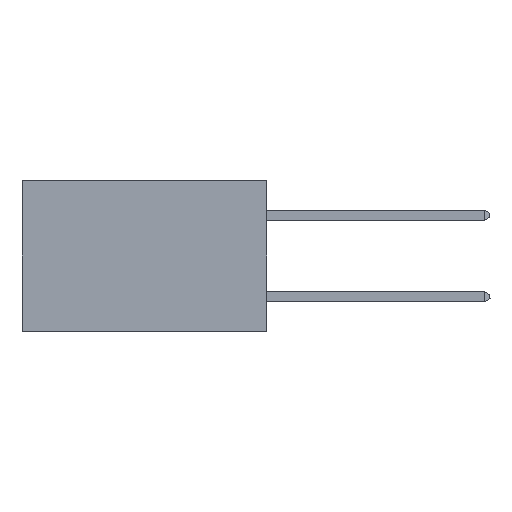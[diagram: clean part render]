
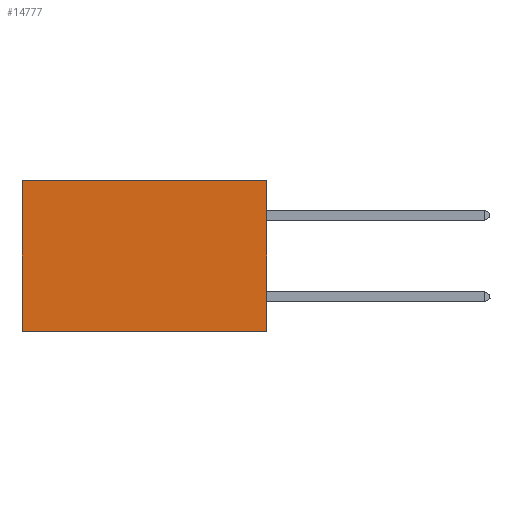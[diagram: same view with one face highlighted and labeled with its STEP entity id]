
A CAD part, left-side view. The second image highlights one B-rep face of the part: STEP entity #14777.
In plain terms, the highlighted planar face has unit normal (-1, 0, 0).
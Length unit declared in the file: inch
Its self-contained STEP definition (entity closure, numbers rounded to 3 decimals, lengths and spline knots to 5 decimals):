
#618 = ORIENTED_EDGE ( 'NONE', *, *, #17312, .T. ) ;
#1189 = VECTOR ( 'NONE', #5908, 39.37008 ) ;
#1414 = CARTESIAN_POINT ( 'NONE',  ( 0.2875, 0.6, 0. ) ) ;
#3554 = VERTEX_POINT ( 'NONE', #24488 ) ;
#5908 = DIRECTION ( 'NONE',  ( 0., 1., 0. ) ) ;
#6450 = FACE_OUTER_BOUND ( 'NONE', #19353, .T. ) ;
#6460 = AXIS2_PLACEMENT_3D ( 'NONE', #15453, #22095, #24395 ) ;
#6669 = LINE ( 'NONE', #29387, #25458 ) ;
#7198 = ORIENTED_EDGE ( 'NONE', *, *, #25629, .T. ) ;
#7609 = VERTEX_POINT ( 'NONE', #23046 ) ;
#7799 = EDGE_CURVE ( 'NONE', #15069, #3554, #20726, .T. ) ;
#9497 = VECTOR ( 'NONE', #23343, 39.37008 ) ;
#10221 = LINE ( 'NONE', #22847, #9497 ) ;
#14090 = DIRECTION ( 'NONE',  ( 0., 0., -1. ) ) ;
#14777 = ADVANCED_FACE ( 'NONE', ( #6450 ), #29092, .F. ) ;
#15069 = VERTEX_POINT ( 'NONE', #26815 ) ;
#15453 = CARTESIAN_POINT ( 'NONE',  ( 0.2875, 0., 0. ) ) ;
#17312 = EDGE_CURVE ( 'NONE', #15069, #22805, #10221, .T. ) ;
#17815 = DIRECTION ( 'NONE',  ( 0., 0., -1. ) ) ;
#18461 = EDGE_CURVE ( 'NONE', #3554, #7609, #23573, .T. ) ;
#19353 = EDGE_LOOP ( 'NONE', ( #7198, #27400, #26225, #618 ) ) ;
#19659 = CARTESIAN_POINT ( 'NONE',  ( 0.2875, 0., -0.37 ) ) ;
#20726 = LINE ( 'NONE', #23398, #29278 ) ;
#22095 = DIRECTION ( 'NONE',  ( 1., 0., 0. ) ) ;
#22805 = VERTEX_POINT ( 'NONE', #1414 ) ;
#22847 = CARTESIAN_POINT ( 'NONE',  ( 0.2875, 0., 0. ) ) ;
#23046 = CARTESIAN_POINT ( 'NONE',  ( 0.2875, 0.6, -0.37 ) ) ;
#23343 = DIRECTION ( 'NONE',  ( 0., 1., 0. ) ) ;
#23398 = CARTESIAN_POINT ( 'NONE',  ( 0.2875, 0., 0. ) ) ;
#23573 = LINE ( 'NONE', #19659, #1189 ) ;
#24395 = DIRECTION ( 'NONE',  ( 0., 0., -1. ) ) ;
#24488 = CARTESIAN_POINT ( 'NONE',  ( 0.2875, 0., -0.37 ) ) ;
#25458 = VECTOR ( 'NONE', #17815, 39.37008 ) ;
#25629 = EDGE_CURVE ( 'NONE', #22805, #7609, #6669, .T. ) ;
#26225 = ORIENTED_EDGE ( 'NONE', *, *, #7799, .F. ) ;
#26815 = CARTESIAN_POINT ( 'NONE',  ( 0.2875, 0., 0. ) ) ;
#27400 = ORIENTED_EDGE ( 'NONE', *, *, #18461, .F. ) ;
#29092 = PLANE ( 'NONE',  #6460 ) ;
#29278 = VECTOR ( 'NONE', #14090, 39.37008 ) ;
#29387 = CARTESIAN_POINT ( 'NONE',  ( 0.2875, 0.6, 0. ) ) ;
